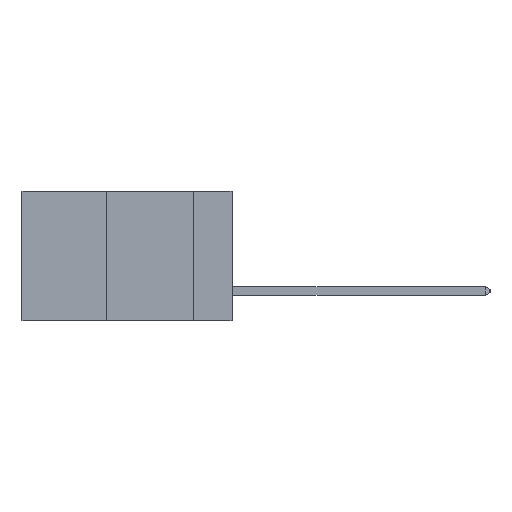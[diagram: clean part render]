
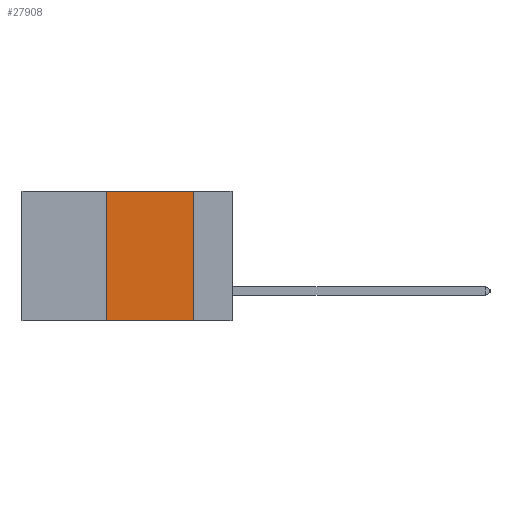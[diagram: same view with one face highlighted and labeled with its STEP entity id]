
A CAD part, left-side view. The second image highlights one B-rep face of the part: STEP entity #27908.
In plain terms, the highlighted planar face has unit normal (-1, 0, 0).
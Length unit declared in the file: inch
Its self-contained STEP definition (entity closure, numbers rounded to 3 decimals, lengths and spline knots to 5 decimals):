
#717 = EDGE_CURVE ( 'NONE', #26912, #17001, #27255, .T. ) ;
#3132 = AXIS2_PLACEMENT_3D ( 'NONE', #18385, #27205, #14005 ) ;
#4273 = CARTESIAN_POINT ( 'NONE',  ( 0., 0.6, 0. ) ) ;
#4551 = CARTESIAN_POINT ( 'NONE',  ( 0., 0.6, -0.37 ) ) ;
#5384 = EDGE_CURVE ( 'NONE', #26912, #9099, #15324, .T. ) ;
#6347 = ORIENTED_EDGE ( 'NONE', *, *, #23100, .F. ) ;
#6635 = ORIENTED_EDGE ( 'NONE', *, *, #5384, .F. ) ;
#7883 = FACE_OUTER_BOUND ( 'NONE', #16939, .T. ) ;
#8741 = ORIENTED_EDGE ( 'NONE', *, *, #11551, .F. ) ;
#9099 = VERTEX_POINT ( 'NONE', #12970 ) ;
#9300 = VECTOR ( 'NONE', #20261, 39.37008 ) ;
#9542 = LINE ( 'NONE', #25674, #14862 ) ;
#11551 = EDGE_CURVE ( 'NONE', #9099, #23657, #21231, .T. ) ;
#11711 = PLANE ( 'NONE',  #3132 ) ;
#11782 = CARTESIAN_POINT ( 'NONE',  ( 0., 0.36, -0.37 ) ) ;
#12970 = CARTESIAN_POINT ( 'NONE',  ( 0., 0.36, 0. ) ) ;
#14005 = DIRECTION ( 'NONE',  ( 0., 0., -1. ) ) ;
#14603 = VECTOR ( 'NONE', #18219, 39.37008 ) ;
#14806 = DIRECTION ( 'NONE',  ( 0., -1., 0. ) ) ;
#14844 = VECTOR ( 'NONE', #14806, 39.37008 ) ;
#14862 = VECTOR ( 'NONE', #27856, 39.37008 ) ;
#15324 = LINE ( 'NONE', #18057, #14603 ) ;
#16939 = EDGE_LOOP ( 'NONE', ( #6347, #8741, #6635, #17907 ) ) ;
#17001 = VERTEX_POINT ( 'NONE', #22917 ) ;
#17907 = ORIENTED_EDGE ( 'NONE', *, *, #717, .T. ) ;
#18057 = CARTESIAN_POINT ( 'NONE',  ( 0., 0.36, 0. ) ) ;
#18219 = DIRECTION ( 'NONE',  ( 0., 0., 1. ) ) ;
#18385 = CARTESIAN_POINT ( 'NONE',  ( 0., 0.6, 0. ) ) ;
#20261 = DIRECTION ( 'NONE',  ( 0., -1., 0. ) ) ;
#20860 = CARTESIAN_POINT ( 'NONE',  ( 0., 0.11, 0. ) ) ;
#21231 = LINE ( 'NONE', #4273, #9300 ) ;
#22917 = CARTESIAN_POINT ( 'NONE',  ( 0., 0.11, -0.37 ) ) ;
#23100 = EDGE_CURVE ( 'NONE', #23657, #17001, #9542, .T. ) ;
#23657 = VERTEX_POINT ( 'NONE', #20860 ) ;
#25674 = CARTESIAN_POINT ( 'NONE',  ( 0., 0.11, 0. ) ) ;
#26912 = VERTEX_POINT ( 'NONE', #11782 ) ;
#27205 = DIRECTION ( 'NONE',  ( 1., 0., 0. ) ) ;
#27255 = LINE ( 'NONE', #4551, #14844 ) ;
#27856 = DIRECTION ( 'NONE',  ( 0., 0., -1. ) ) ;
#27908 = ADVANCED_FACE ( 'NONE', ( #7883 ), #11711, .F. ) ;
